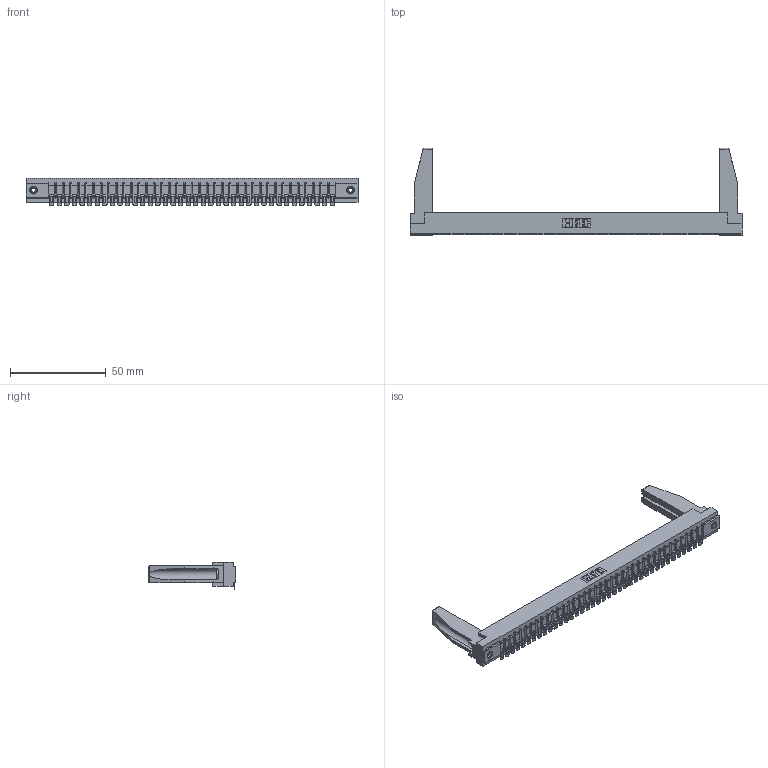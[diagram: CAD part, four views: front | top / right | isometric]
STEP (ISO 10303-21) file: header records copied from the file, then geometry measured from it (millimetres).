
FILE_DESCRIPTION (( 'STEP AP203' ), '1' );
FILE_NAME ('307-038-454-178.STEP', '2020-09-29T06:41:51', ( '' ), ( '' ), 'SwSTEP 2.0', 'SolidWorks 2020', '' );
FILE_SCHEMA (( 'CONFIG_CONTROL_DESIGN' ));
Length unit declared in the file: inch
Products named in the file (5): 307-290-002_554; 345-250-001_345-250-001-102; 307 Part_.156 Dia Mounting Holes; 307-038-454-178; 307-220-078
Assembly tree (43 placements, depth 2):
  307-038-454-178
    307 Part_.156 Dia Mounting Holes
    307-290-002_554  x38
    307-220-078  x2
    345-250-001_345-250-001-102  x2
Bounding box: 173.58 x 45.72 x 14.52 mm (x, y, z)
Volume: 22552.8 mm3; surface area: 27220 mm2
Topology: 43 solids, 43 shells, 3365 faces, 10267 edges, 6730 vertices
Faces by surface type: plane 1902, cylinder 1369, sphere 78, cone 12, torus 4
Entity records: 36474 total; most frequent: CARTESIAN_POINT 6152, ORIENTED_EDGE 6098, DIRECTION 5941, EDGE_CURVE 3049, VECTOR 2331, LINE 2331, VERTEX_POINT 1974, AXIS2_PLACEMENT_3D 1805
